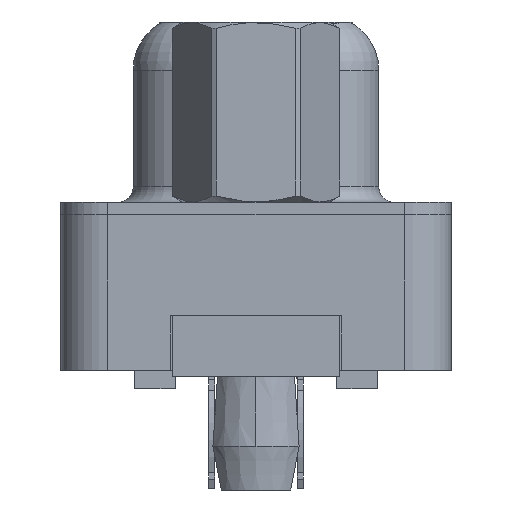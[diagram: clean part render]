
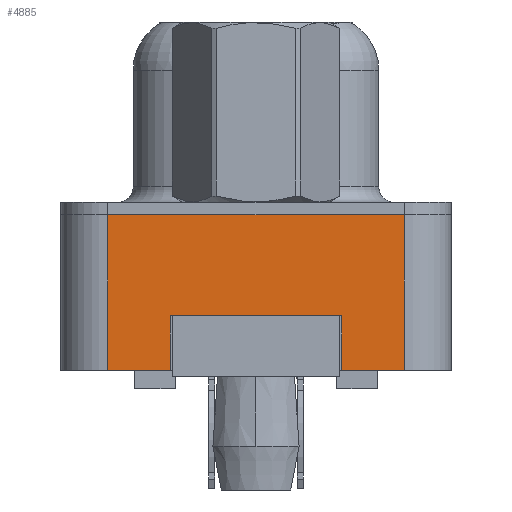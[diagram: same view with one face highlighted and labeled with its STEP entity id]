
A CAD part, left-side view. The second image highlights one B-rep face of the part: STEP entity #4885.
In plain terms, the highlighted planar face has unit normal (-1, 0, 0).
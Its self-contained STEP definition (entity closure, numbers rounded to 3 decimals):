
#386 = LINE ( 'NONE', #24560, #6298 ) ;
#700 = CARTESIAN_POINT ( 'NONE',  ( -2.995, -4.775, -5. ) ) ;
#985 = EDGE_CURVE ( 'NONE', #7225, #13158, #386, .T. ) ;
#1279 = CARTESIAN_POINT ( 'NONE',  ( -2.995, 2.75, -3.25 ) ) ;
#1907 = CARTESIAN_POINT ( 'NONE',  ( -2.995, -2.75, -3.25 ) ) ;
#1998 = VERTEX_POINT ( 'NONE', #22580 ) ;
#2778 = DIRECTION ( 'NONE',  ( 0., -1., 0. ) ) ;
#3640 = EDGE_CURVE ( 'NONE', #7753, #13827, #8126, .T. ) ;
#3751 = DIRECTION ( 'NONE',  ( 0., -1., 0. ) ) ;
#4265 = ORIENTED_EDGE ( 'NONE', *, *, #3640, .T. ) ;
#4416 = CARTESIAN_POINT ( 'NONE',  ( -2.995, -4.775, 0. ) ) ;
#4561 = CARTESIAN_POINT ( 'NONE',  ( -2.995, 4.775, -5. ) ) ;
#4885 = ADVANCED_FACE ( 'NONE', ( #23343 ), #23465, .T. ) ;
#6203 = CARTESIAN_POINT ( 'NONE',  ( -2.995, 2.75, -3.25 ) ) ;
#6298 = VECTOR ( 'NONE', #6442, 1000. ) ;
#6442 = DIRECTION ( 'NONE',  ( 0., 0., -1. ) ) ;
#6505 = VERTEX_POINT ( 'NONE', #24596 ) ;
#6781 = EDGE_CURVE ( 'NONE', #22237, #10205, #22702, .T. ) ;
#7081 = EDGE_CURVE ( 'NONE', #6505, #10205, #23476, .T. ) ;
#7225 = VERTEX_POINT ( 'NONE', #1907 ) ;
#7312 = ORIENTED_EDGE ( 'NONE', *, *, #17493, .T. ) ;
#7753 = VERTEX_POINT ( 'NONE', #19929 ) ;
#7819 = DIRECTION ( 'NONE',  ( 0., 0., -1. ) ) ;
#8126 = LINE ( 'NONE', #16213, #25567 ) ;
#8700 = CARTESIAN_POINT ( 'NONE',  ( -2.995, 2.75, -5. ) ) ;
#9050 = ORIENTED_EDGE ( 'NONE', *, *, #23815, .F. ) ;
#9434 = CARTESIAN_POINT ( 'NONE',  ( -2.995, -4.775, -5. ) ) ;
#9877 = EDGE_CURVE ( 'NONE', #7225, #1998, #22229, .T. ) ;
#10205 = VERTEX_POINT ( 'NONE', #22064 ) ;
#11619 = ORIENTED_EDGE ( 'NONE', *, *, #6781, .F. ) ;
#11847 = EDGE_CURVE ( 'NONE', #1998, #13827, #20003, .T. ) ;
#13008 = ORIENTED_EDGE ( 'NONE', *, *, #985, .T. ) ;
#13158 = VERTEX_POINT ( 'NONE', #20432 ) ;
#13827 = VERTEX_POINT ( 'NONE', #8700 ) ;
#14285 = DIRECTION ( 'NONE',  ( 0., 1., 0. ) ) ;
#15014 = VECTOR ( 'NONE', #2778, 1000. ) ;
#15801 = ORIENTED_EDGE ( 'NONE', *, *, #9877, .F. ) ;
#16213 = CARTESIAN_POINT ( 'NONE',  ( -2.995, -4.775, -5. ) ) ;
#16693 = LINE ( 'NONE', #700, #15014 ) ;
#16899 = LINE ( 'NONE', #4561, #19767 ) ;
#17493 = EDGE_CURVE ( 'NONE', #13158, #6505, #16693, .T. ) ;
#18589 = DIRECTION ( 'NONE',  ( 0., -1., 0. ) ) ;
#18598 = DIRECTION ( 'NONE',  ( 0., 0., 1. ) ) ;
#19275 = VECTOR ( 'NONE', #18589, 1000. ) ;
#19767 = VECTOR ( 'NONE', #18598, 1000. ) ;
#19929 = CARTESIAN_POINT ( 'NONE',  ( -2.995, 4.775, -5. ) ) ;
#20003 = LINE ( 'NONE', #1279, #23335 ) ;
#20432 = CARTESIAN_POINT ( 'NONE',  ( -2.995, -2.75, -5. ) ) ;
#21219 = CARTESIAN_POINT ( 'NONE',  ( -2.995, -4.775, -5. ) ) ;
#21472 = DIRECTION ( 'NONE',  ( -1., 0., 0. ) ) ;
#21557 = ORIENTED_EDGE ( 'NONE', *, *, #7081, .T. ) ;
#22064 = CARTESIAN_POINT ( 'NONE',  ( -2.995, -4.775, 0. ) ) ;
#22229 = LINE ( 'NONE', #6203, #24436 ) ;
#22237 = VERTEX_POINT ( 'NONE', #25510 ) ;
#22285 = EDGE_LOOP ( 'NONE', ( #13008, #7312, #21557, #11619, #9050, #4265, #26037, #15801 ) ) ;
#22580 = CARTESIAN_POINT ( 'NONE',  ( -2.995, 2.75, -3.25 ) ) ;
#22702 = LINE ( 'NONE', #4416, #19275 ) ;
#23335 = VECTOR ( 'NONE', #7819, 1000. ) ;
#23343 = FACE_OUTER_BOUND ( 'NONE', #22285, .T. ) ;
#23465 = PLANE ( 'NONE',  #23473 ) ;
#23473 = AXIS2_PLACEMENT_3D ( 'NONE', #21219, #21472, #25559 ) ;
#23476 = LINE ( 'NONE', #9434, #23949 ) ;
#23815 = EDGE_CURVE ( 'NONE', #7753, #22237, #16899, .T. ) ;
#23949 = VECTOR ( 'NONE', #23990, 1000. ) ;
#23990 = DIRECTION ( 'NONE',  ( 0., 0., 1. ) ) ;
#24436 = VECTOR ( 'NONE', #14285, 1000. ) ;
#24560 = CARTESIAN_POINT ( 'NONE',  ( -2.995, -2.75, -3.25 ) ) ;
#24596 = CARTESIAN_POINT ( 'NONE',  ( -2.995, -4.775, -5. ) ) ;
#25510 = CARTESIAN_POINT ( 'NONE',  ( -2.995, 4.775, 0. ) ) ;
#25559 = DIRECTION ( 'NONE',  ( 0., 0., 1. ) ) ;
#25567 = VECTOR ( 'NONE', #3751, 1000. ) ;
#26037 = ORIENTED_EDGE ( 'NONE', *, *, #11847, .F. ) ;
